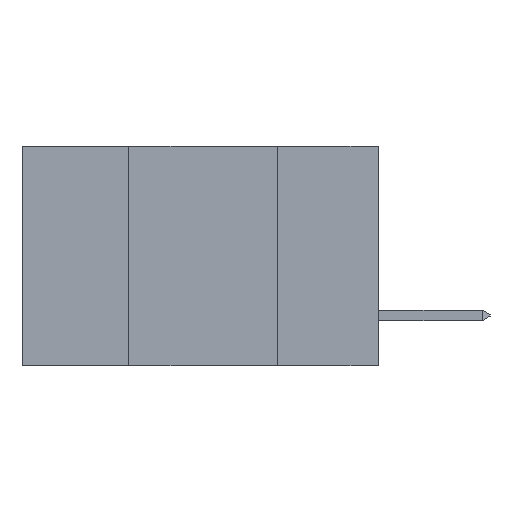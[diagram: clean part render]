
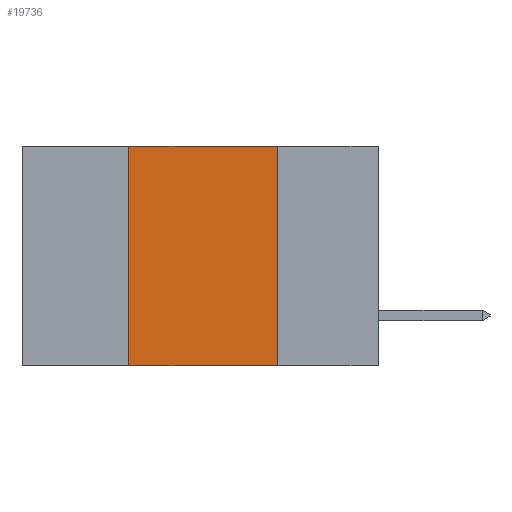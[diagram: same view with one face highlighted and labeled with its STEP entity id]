
A CAD part, left-side view. The second image highlights one B-rep face of the part: STEP entity #19736.
In plain terms, the highlighted planar face has unit normal (-1, 0, 0).
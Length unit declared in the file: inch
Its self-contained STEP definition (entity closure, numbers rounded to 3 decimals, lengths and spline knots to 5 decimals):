
#729 = CARTESIAN_POINT ( 'NONE',  ( 0., 0.42, -0.37 ) ) ;
#2414 = FACE_OUTER_BOUND ( 'NONE', #11710, .T. ) ;
#2751 = DIRECTION ( 'NONE',  ( 0., -1., 0. ) ) ;
#2865 = LINE ( 'NONE', #19505, #15431 ) ;
#3825 = ORIENTED_EDGE ( 'NONE', *, *, #12412, .F. ) ;
#5164 = LINE ( 'NONE', #15177, #18143 ) ;
#5247 = CARTESIAN_POINT ( 'NONE',  ( 0., 0.17, 0. ) ) ;
#5481 = EDGE_CURVE ( 'NONE', #14816, #18231, #5164, .T. ) ;
#7050 = ORIENTED_EDGE ( 'NONE', *, *, #16250, .F. ) ;
#7179 = LINE ( 'NONE', #17067, #19537 ) ;
#7333 = VECTOR ( 'NONE', #2751, 39.37008 ) ;
#7786 = CARTESIAN_POINT ( 'NONE',  ( 0., 0.6, 0. ) ) ;
#7823 = LINE ( 'NONE', #19038, #7333 ) ;
#8203 = DIRECTION ( 'NONE',  ( 0., 0., -1. ) ) ;
#8536 = CARTESIAN_POINT ( 'NONE',  ( 0., 0.17, -0.37 ) ) ;
#8891 = DIRECTION ( 'NONE',  ( 0., 0., 1. ) ) ;
#9376 = DIRECTION ( 'NONE',  ( 0., 0., -1. ) ) ;
#9844 = VERTEX_POINT ( 'NONE', #19211 ) ;
#10084 = AXIS2_PLACEMENT_3D ( 'NONE', #7786, #19084, #9376 ) ;
#11710 = EDGE_LOOP ( 'NONE', ( #14894, #3825, #7050, #16155 ) ) ;
#12410 = DIRECTION ( 'NONE',  ( 0., -1., 0. ) ) ;
#12412 = EDGE_CURVE ( 'NONE', #9844, #15279, #7823, .T. ) ;
#13136 = EDGE_CURVE ( 'NONE', #15279, #18231, #2865, .T. ) ;
#14247 = PLANE ( 'NONE',  #10084 ) ;
#14816 = VERTEX_POINT ( 'NONE', #729 ) ;
#14894 = ORIENTED_EDGE ( 'NONE', *, *, #13136, .F. ) ;
#15177 = CARTESIAN_POINT ( 'NONE',  ( 0., 0.6, -0.37 ) ) ;
#15279 = VERTEX_POINT ( 'NONE', #5247 ) ;
#15431 = VECTOR ( 'NONE', #8203, 39.37008 ) ;
#16155 = ORIENTED_EDGE ( 'NONE', *, *, #5481, .T. ) ;
#16250 = EDGE_CURVE ( 'NONE', #14816, #9844, #7179, .T. ) ;
#17067 = CARTESIAN_POINT ( 'NONE',  ( 0., 0.42, 0. ) ) ;
#18143 = VECTOR ( 'NONE', #12410, 39.37008 ) ;
#18231 = VERTEX_POINT ( 'NONE', #8536 ) ;
#19038 = CARTESIAN_POINT ( 'NONE',  ( 0., 0.6, 0. ) ) ;
#19084 = DIRECTION ( 'NONE',  ( 1., 0., 0. ) ) ;
#19211 = CARTESIAN_POINT ( 'NONE',  ( 0., 0.42, 0. ) ) ;
#19505 = CARTESIAN_POINT ( 'NONE',  ( 0., 0.17, 0. ) ) ;
#19537 = VECTOR ( 'NONE', #8891, 39.37008 ) ;
#19736 = ADVANCED_FACE ( 'NONE', ( #2414 ), #14247, .F. ) ;
